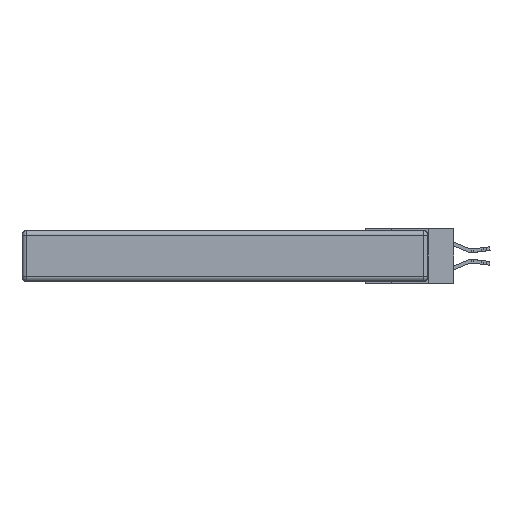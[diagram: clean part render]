
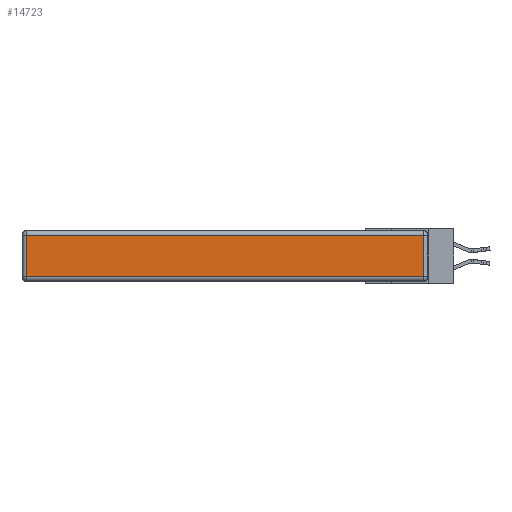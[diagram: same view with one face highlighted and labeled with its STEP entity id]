
A CAD part, left-side view. The second image highlights one B-rep face of the part: STEP entity #14723.
In plain terms, the highlighted planar face has unit normal (-1, 0, 0).
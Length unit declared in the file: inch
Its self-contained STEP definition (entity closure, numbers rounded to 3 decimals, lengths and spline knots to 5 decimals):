
#1061 = CARTESIAN_POINT ( 'NONE',  ( 0., 0.03, -0.343 ) ) ;
#1152 = LINE ( 'NONE', #5209, #22004 ) ;
#1832 = VERTEX_POINT ( 'NONE', #18125 ) ;
#2926 = LINE ( 'NONE', #25805, #32419 ) ;
#5209 = CARTESIAN_POINT ( 'NONE',  ( 0., 2.75, -0.03 ) ) ;
#5230 = EDGE_LOOP ( 'NONE', ( #32421, #13811, #26505, #20379 ) ) ;
#6417 = CARTESIAN_POINT ( 'NONE',  ( 0., 0.03, -0.313 ) ) ;
#8671 = DIRECTION ( 'NONE',  ( 0., -1., 0. ) ) ;
#9746 = EDGE_CURVE ( 'NONE', #19016, #21826, #31797, .T. ) ;
#10054 = VERTEX_POINT ( 'NONE', #32066 ) ;
#10978 = LINE ( 'NONE', #1061, #32210 ) ;
#11060 = CARTESIAN_POINT ( 'NONE',  ( 0., 2.72, -0.313 ) ) ;
#12513 = VECTOR ( 'NONE', #8671, 39.37008 ) ;
#13811 = ORIENTED_EDGE ( 'NONE', *, *, #25019, .T. ) ;
#14723 = ADVANCED_FACE ( 'NONE', ( #30963 ), #29103, .T. ) ;
#16984 = CARTESIAN_POINT ( 'NONE',  ( 0., 0., -0.343 ) ) ;
#17904 = DIRECTION ( 'NONE',  ( 0., 0., -1. ) ) ;
#18125 = CARTESIAN_POINT ( 'NONE',  ( 0., 2.72, -0.03 ) ) ;
#18328 = DIRECTION ( 'NONE',  ( 0., 0., 1. ) ) ;
#19016 = VERTEX_POINT ( 'NONE', #11060 ) ;
#19290 = EDGE_CURVE ( 'NONE', #10054, #1832, #1152, .T. ) ;
#19393 = DIRECTION ( 'NONE',  ( -1., 0., 0. ) ) ;
#20379 = ORIENTED_EDGE ( 'NONE', *, *, #22083, .T. ) ;
#21826 = VERTEX_POINT ( 'NONE', #6417 ) ;
#22004 = VECTOR ( 'NONE', #22450, 39.37008 ) ;
#22083 = EDGE_CURVE ( 'NONE', #1832, #19016, #2926, .T. ) ;
#22450 = DIRECTION ( 'NONE',  ( 0., 1., 0. ) ) ;
#25019 = EDGE_CURVE ( 'NONE', #21826, #10054, #10978, .T. ) ;
#25805 = CARTESIAN_POINT ( 'NONE',  ( 0., 2.72, -0.343 ) ) ;
#26505 = ORIENTED_EDGE ( 'NONE', *, *, #19290, .T. ) ;
#28708 = CARTESIAN_POINT ( 'NONE',  ( 0., 0., -0.313 ) ) ;
#29103 = PLANE ( 'NONE',  #30648 ) ;
#29314 = DIRECTION ( 'NONE',  ( 0., 0., 1. ) ) ;
#30648 = AXIS2_PLACEMENT_3D ( 'NONE', #16984, #19393, #29314 ) ;
#30963 = FACE_OUTER_BOUND ( 'NONE', #5230, .T. ) ;
#31797 = LINE ( 'NONE', #28708, #12513 ) ;
#32066 = CARTESIAN_POINT ( 'NONE',  ( 0., 0.03, -0.03 ) ) ;
#32210 = VECTOR ( 'NONE', #18328, 39.37008 ) ;
#32419 = VECTOR ( 'NONE', #17904, 39.37008 ) ;
#32421 = ORIENTED_EDGE ( 'NONE', *, *, #9746, .T. ) ;
